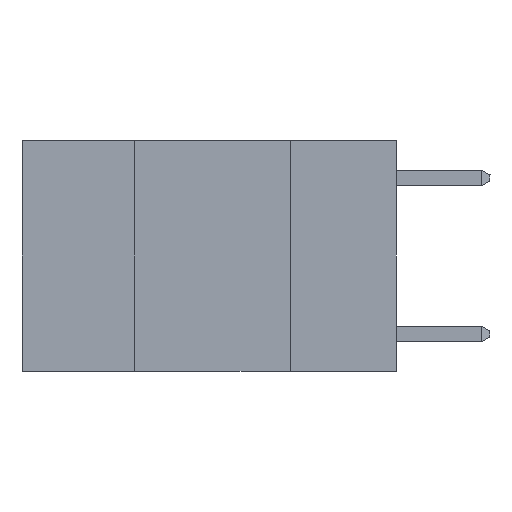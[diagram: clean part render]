
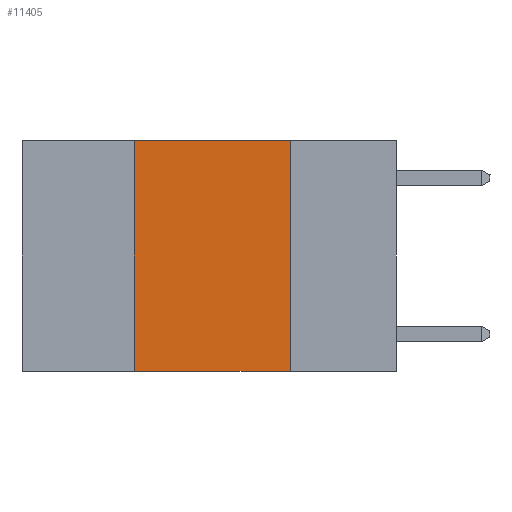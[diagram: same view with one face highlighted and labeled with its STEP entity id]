
A CAD part, left-side view. The second image highlights one B-rep face of the part: STEP entity #11405.
In plain terms, the highlighted planar face has unit normal (-1, 0, 0).
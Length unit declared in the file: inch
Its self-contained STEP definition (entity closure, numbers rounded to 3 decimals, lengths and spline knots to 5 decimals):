
#41 = VECTOR ( 'NONE', #13818, 39.37008 ) ;
#92 = DIRECTION ( 'NONE',  ( 1., 0., 0. ) ) ;
#317 = CARTESIAN_POINT ( 'NONE',  ( 0., 0.17, 0. ) ) ;
#911 = EDGE_CURVE ( 'NONE', #21446, #20111, #13064, .T. ) ;
#1908 = DIRECTION ( 'NONE',  ( 0., 0., 1. ) ) ;
#2435 = VECTOR ( 'NONE', #22900, 39.37008 ) ;
#2633 = CARTESIAN_POINT ( 'NONE',  ( 0., 0.17, -0.37 ) ) ;
#2882 = VECTOR ( 'NONE', #9351, 39.37008 ) ;
#2910 = EDGE_LOOP ( 'NONE', ( #20180, #20651, #20678, #21898 ) ) ;
#2925 = CARTESIAN_POINT ( 'NONE',  ( 0., 0.17, 0. ) ) ;
#3178 = VECTOR ( 'NONE', #1908, 39.37008 ) ;
#3255 = VERTEX_POINT ( 'NONE', #17206 ) ;
#6481 = CARTESIAN_POINT ( 'NONE',  ( 0., 0.42, 0. ) ) ;
#6713 = EDGE_CURVE ( 'NONE', #3255, #10463, #22565, .T. ) ;
#8877 = LINE ( 'NONE', #24435, #3178 ) ;
#9351 = DIRECTION ( 'NONE',  ( 0., -1., 0. ) ) ;
#9736 = CARTESIAN_POINT ( 'NONE',  ( 0., 0.6, 0. ) ) ;
#10463 = VERTEX_POINT ( 'NONE', #2633 ) ;
#11405 = ADVANCED_FACE ( 'NONE', ( #19378 ), #21032, .F. ) ;
#11661 = CARTESIAN_POINT ( 'NONE',  ( 0., 0.6, 0. ) ) ;
#11701 = CARTESIAN_POINT ( 'NONE',  ( 0., 0.6, -0.37 ) ) ;
#13064 = LINE ( 'NONE', #9736, #2882 ) ;
#13605 = DIRECTION ( 'NONE',  ( 0., 0., -1. ) ) ;
#13818 = DIRECTION ( 'NONE',  ( 0., 0., -1. ) ) ;
#13841 = AXIS2_PLACEMENT_3D ( 'NONE', #11661, #92, #13605 ) ;
#14839 = LINE ( 'NONE', #317, #41 ) ;
#17206 = CARTESIAN_POINT ( 'NONE',  ( 0., 0.42, -0.37 ) ) ;
#17752 = EDGE_CURVE ( 'NONE', #3255, #21446, #8877, .T. ) ;
#17886 = EDGE_CURVE ( 'NONE', #20111, #10463, #14839, .T. ) ;
#19378 = FACE_OUTER_BOUND ( 'NONE', #2910, .T. ) ;
#20111 = VERTEX_POINT ( 'NONE', #2925 ) ;
#20180 = ORIENTED_EDGE ( 'NONE', *, *, #17886, .F. ) ;
#20651 = ORIENTED_EDGE ( 'NONE', *, *, #911, .F. ) ;
#20678 = ORIENTED_EDGE ( 'NONE', *, *, #17752, .F. ) ;
#21032 = PLANE ( 'NONE',  #13841 ) ;
#21446 = VERTEX_POINT ( 'NONE', #6481 ) ;
#21898 = ORIENTED_EDGE ( 'NONE', *, *, #6713, .T. ) ;
#22565 = LINE ( 'NONE', #11701, #2435 ) ;
#22900 = DIRECTION ( 'NONE',  ( 0., -1., 0. ) ) ;
#24435 = CARTESIAN_POINT ( 'NONE',  ( 0., 0.42, 0. ) ) ;
